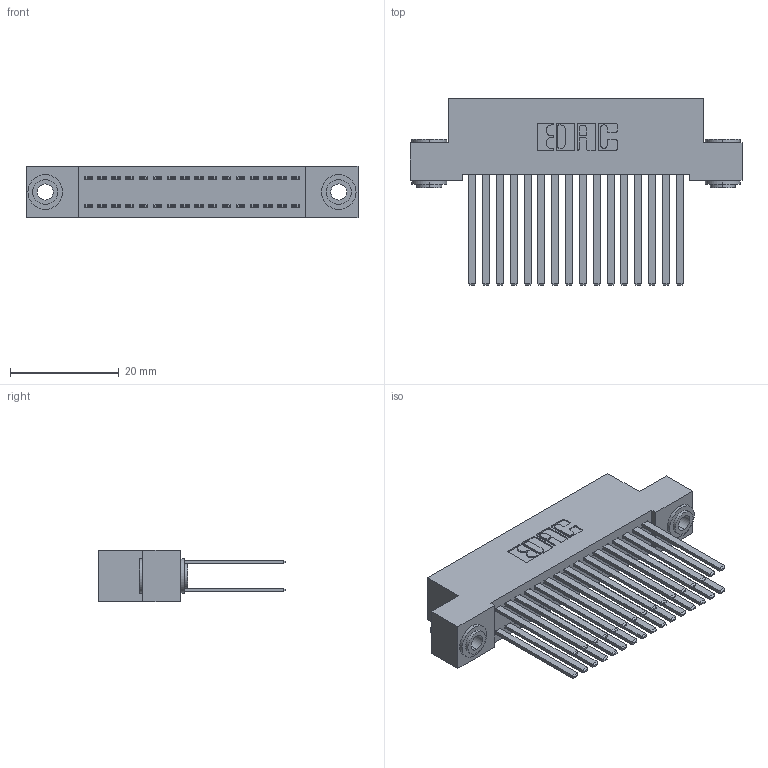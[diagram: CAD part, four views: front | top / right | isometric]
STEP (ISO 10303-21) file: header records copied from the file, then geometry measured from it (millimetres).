
FILE_DESCRIPTION (( 'STEP AP203' ), '1' );
FILE_NAME ('342-032-544-203.STEP', '2018-08-11T17:12:01', ( '' ), ( '' ), 'SwSTEP 2.0', 'SolidWorks 2016', '' );
FILE_SCHEMA (( 'CONFIG_CONTROL_DESIGN' ));
Length unit declared in the file: inch
Products named in the file (4): 342 Part_.156 TH; 345-292-001_345-293-144; 342-250-002_345-250-002-102; 342-032-544-203
Assembly tree (35 placements, depth 2):
  342-032-544-203
    342 Part_.156 TH
    345-292-001_345-293-144  x32
    342-250-002_345-250-002-102  x2
Bounding box: 60.96 x 34.3 x 9.4 mm (x, y, z)
Volume: 5825.6 mm3; surface area: 10298.3 mm2
Topology: 35 solids, 35 shells, 1620 faces, 4759 edges, 3126 vertices
Faces by surface type: plane 1100, cylinder 512, cone 8
Entity records: 13990 total; most frequent: CARTESIAN_POINT 2321, ORIENTED_EDGE 2250, DIRECTION 2059, EDGE_CURVE 1125, VECTOR 977, LINE 977, VERTEX_POINT 746, AXIS2_PLACEMENT_3D 541
